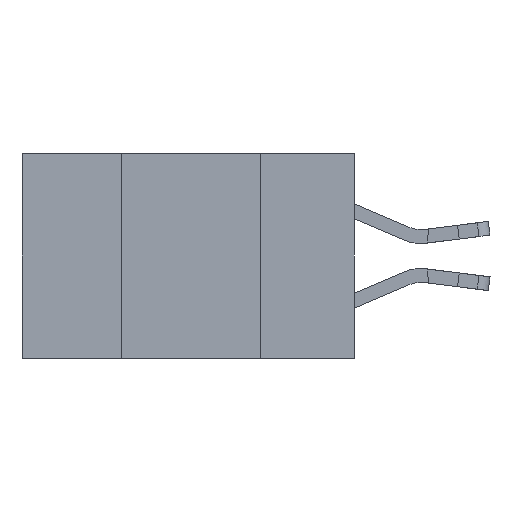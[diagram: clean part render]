
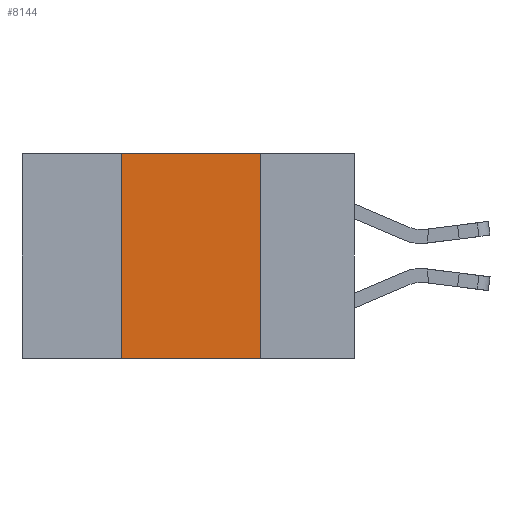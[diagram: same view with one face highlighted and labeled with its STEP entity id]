
A CAD part, left-side view. The second image highlights one B-rep face of the part: STEP entity #8144.
In plain terms, the highlighted planar face has unit normal (-1, 0, 0).
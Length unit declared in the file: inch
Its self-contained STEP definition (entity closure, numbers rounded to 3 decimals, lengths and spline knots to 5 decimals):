
#113 = CARTESIAN_POINT ( 'NONE',  ( 0., 0.17, -0.37 ) ) ;
#673 = LINE ( 'NONE', #8844, #8329 ) ;
#712 = VERTEX_POINT ( 'NONE', #4837 ) ;
#779 = LINE ( 'NONE', #3514, #10936 ) ;
#1622 = VERTEX_POINT ( 'NONE', #2871 ) ;
#1791 = EDGE_LOOP ( 'NONE', ( #8535, #12563, #10005, #10176 ) ) ;
#1978 = VERTEX_POINT ( 'NONE', #113 ) ;
#2035 = DIRECTION ( 'NONE',  ( 0., 0., -1. ) ) ;
#2140 = DIRECTION ( 'NONE',  ( 0., 0., 1. ) ) ;
#2871 = CARTESIAN_POINT ( 'NONE',  ( 0., 0.17, 0. ) ) ;
#3233 = EDGE_CURVE ( 'NONE', #712, #1622, #779, .T. ) ;
#3514 = CARTESIAN_POINT ( 'NONE',  ( 0., 0.6, 0. ) ) ;
#4405 = LINE ( 'NONE', #10110, #7435 ) ;
#4457 = CARTESIAN_POINT ( 'NONE',  ( 0., 0.6, 0. ) ) ;
#4492 = VERTEX_POINT ( 'NONE', #7985 ) ;
#4680 = DIRECTION ( 'NONE',  ( 0., -1., 0. ) ) ;
#4837 = CARTESIAN_POINT ( 'NONE',  ( 0., 0.42, 0. ) ) ;
#5588 = EDGE_CURVE ( 'NONE', #4492, #712, #4405, .T. ) ;
#5602 = DIRECTION ( 'NONE',  ( 0., 0., -1. ) ) ;
#6086 = FACE_OUTER_BOUND ( 'NONE', #1791, .T. ) ;
#6460 = DIRECTION ( 'NONE',  ( 0., -1., 0. ) ) ;
#7435 = VECTOR ( 'NONE', #2140, 39.37008 ) ;
#7985 = CARTESIAN_POINT ( 'NONE',  ( 0., 0.42, -0.37 ) ) ;
#7997 = EDGE_CURVE ( 'NONE', #4492, #1978, #14343, .T. ) ;
#8144 = ADVANCED_FACE ( 'NONE', ( #6086 ), #11313, .F. ) ;
#8329 = VECTOR ( 'NONE', #2035, 39.37008 ) ;
#8535 = ORIENTED_EDGE ( 'NONE', *, *, #10347, .F. ) ;
#8844 = CARTESIAN_POINT ( 'NONE',  ( 0., 0.17, -0.37 ) ) ;
#10005 = ORIENTED_EDGE ( 'NONE', *, *, #5588, .F. ) ;
#10110 = CARTESIAN_POINT ( 'NONE',  ( 0., 0.42, -0.37 ) ) ;
#10176 = ORIENTED_EDGE ( 'NONE', *, *, #7997, .T. ) ;
#10347 = EDGE_CURVE ( 'NONE', #1622, #1978, #673, .T. ) ;
#10565 = VECTOR ( 'NONE', #6460, 39.37008 ) ;
#10936 = VECTOR ( 'NONE', #4680, 39.37008 ) ;
#11313 = PLANE ( 'NONE',  #13856 ) ;
#12447 = DIRECTION ( 'NONE',  ( 1., 0., 0. ) ) ;
#12563 = ORIENTED_EDGE ( 'NONE', *, *, #3233, .F. ) ;
#13856 = AXIS2_PLACEMENT_3D ( 'NONE', #4457, #12447, #5602 ) ;
#14343 = LINE ( 'NONE', #14471, #10565 ) ;
#14471 = CARTESIAN_POINT ( 'NONE',  ( 0., 0.6, -0.37 ) ) ;
